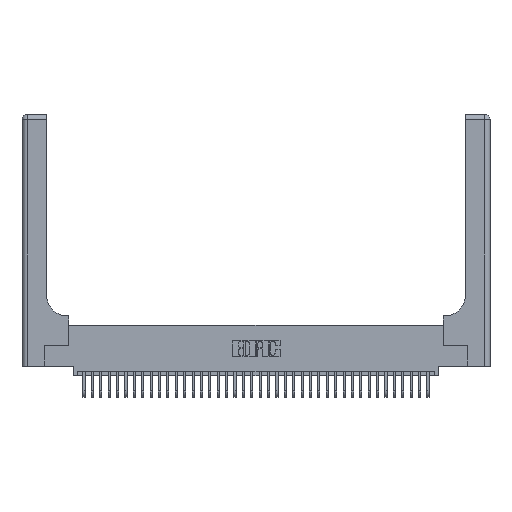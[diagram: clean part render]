
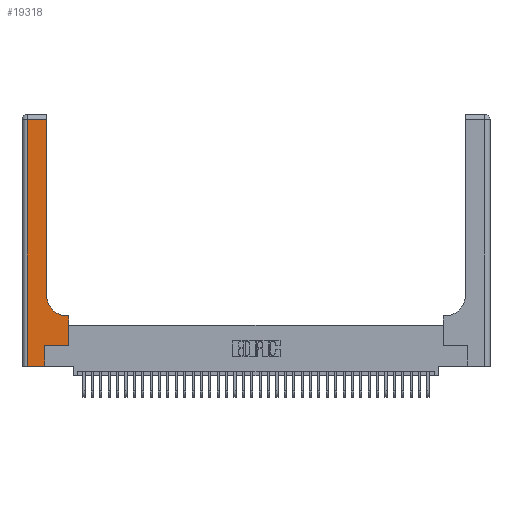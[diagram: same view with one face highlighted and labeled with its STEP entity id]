
A CAD part, top view. The second image highlights one B-rep face of the part: STEP entity #19318.
In plain terms, the highlighted planar face has unit normal (0, 0, 1).
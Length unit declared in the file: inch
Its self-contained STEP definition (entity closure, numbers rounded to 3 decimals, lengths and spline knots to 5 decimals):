
#776 = LINE ( 'NONE', #36630, #22763 ) ;
#889 = VECTOR ( 'NONE', #21785, 39.37008 ) ;
#1633 = VERTEX_POINT ( 'NONE', #10770 ) ;
#1686 = FACE_OUTER_BOUND ( 'NONE', #3178, .T. ) ;
#2050 = ORIENTED_EDGE ( 'NONE', *, *, #23361, .T. ) ;
#2193 = DIRECTION ( 'NONE',  ( -1., 0., 0. ) ) ;
#2312 = DIRECTION ( 'NONE',  ( 0., 0., -1. ) ) ;
#2443 = DIRECTION ( 'NONE',  ( 0., 1., 0. ) ) ;
#2701 = LINE ( 'NONE', #18924, #889 ) ;
#3178 = EDGE_LOOP ( 'NONE', ( #25316, #3786, #7362, #2050, #15601, #27718, #29947, #26872, #20190 ) ) ;
#3778 = VERTEX_POINT ( 'NONE', #33746 ) ;
#3786 = ORIENTED_EDGE ( 'NONE', *, *, #19397, .T. ) ;
#4239 = EDGE_CURVE ( 'NONE', #28799, #34253, #14314, .T. ) ;
#5014 = VERTEX_POINT ( 'NONE', #9779 ) ;
#5049 = CARTESIAN_POINT ( 'NONE',  ( 0.2915, 2.94, 0.37 ) ) ;
#5050 = CARTESIAN_POINT ( 'NONE',  ( 0., 3., 0.37 ) ) ;
#5484 = CARTESIAN_POINT ( 'NONE',  ( 0., 0., 0.37 ) ) ;
#5596 = VERTEX_POINT ( 'NONE', #29403 ) ;
#5608 = VERTEX_POINT ( 'NONE', #12269 ) ;
#7362 = ORIENTED_EDGE ( 'NONE', *, *, #17965, .T. ) ;
#7402 = EDGE_CURVE ( 'NONE', #5014, #5608, #26647, .T. ) ;
#8369 = DIRECTION ( 'NONE',  ( 1., 0., 0. ) ) ;
#8679 = DIRECTION ( 'NONE',  ( 1., 0., 0. ) ) ;
#9344 = DIRECTION ( 'NONE',  ( 0., 1., 0. ) ) ;
#9470 = LINE ( 'NONE', #25890, #30508 ) ;
#9779 = CARTESIAN_POINT ( 'NONE',  ( 0.5585, 0.25, 0.37 ) ) ;
#10365 = DIRECTION ( 'NONE',  ( 0., 1., 0. ) ) ;
#10770 = CARTESIAN_POINT ( 'NONE',  ( 0.5415, 0.6, 0.37 ) ) ;
#11122 = VERTEX_POINT ( 'NONE', #36962 ) ;
#12269 = CARTESIAN_POINT ( 'NONE',  ( 0.5585, 0.6, 0.37 ) ) ;
#13346 = LINE ( 'NONE', #28493, #35201 ) ;
#14314 = LINE ( 'NONE', #21766, #36116 ) ;
#15325 = CARTESIAN_POINT ( 'NONE',  ( 0.5415, 0.85, 0.37 ) ) ;
#15601 = ORIENTED_EDGE ( 'NONE', *, *, #19333, .T. ) ;
#17061 = EDGE_CURVE ( 'NONE', #23232, #5014, #9470, .T. ) ;
#17965 = EDGE_CURVE ( 'NONE', #5596, #11122, #2701, .T. ) ;
#18219 = DIRECTION ( 'NONE',  ( 1., 0., 0. ) ) ;
#18924 = CARTESIAN_POINT ( 'NONE',  ( 0.06, 3., 0.37 ) ) ;
#19011 = VECTOR ( 'NONE', #9344, 39.37008 ) ;
#19014 = LINE ( 'NONE', #30839, #33268 ) ;
#19318 = ADVANCED_FACE ( 'NONE', ( #1686 ), #19497, .F. ) ;
#19333 = EDGE_CURVE ( 'NONE', #3778, #23232, #776, .T. ) ;
#19397 = EDGE_CURVE ( 'NONE', #34253, #5596, #13346, .T. ) ;
#19497 = PLANE ( 'NONE',  #31866 ) ;
#19619 = CARTESIAN_POINT ( 'NONE',  ( 0.2915, 0.85, 0.37 ) ) ;
#20190 = ORIENTED_EDGE ( 'NONE', *, *, #34643, .T. ) ;
#20896 = CARTESIAN_POINT ( 'NONE',  ( 0.5585, 0.25, 0.37 ) ) ;
#21766 = CARTESIAN_POINT ( 'NONE',  ( 0.2915, 3., 0.37 ) ) ;
#21785 = DIRECTION ( 'NONE',  ( 0., -1., 0. ) ) ;
#22364 = DIRECTION ( 'NONE',  ( -1., 0., 0. ) ) ;
#22566 = CIRCLE ( 'NONE', #32774, 0.25 ) ;
#22763 = VECTOR ( 'NONE', #2443, 39.37008 ) ;
#23232 = VERTEX_POINT ( 'NONE', #36202 ) ;
#23361 = EDGE_CURVE ( 'NONE', #11122, #3778, #36904, .T. ) ;
#25316 = ORIENTED_EDGE ( 'NONE', *, *, #4239, .T. ) ;
#25890 = CARTESIAN_POINT ( 'NONE',  ( 0.269, 0.25, 0.37 ) ) ;
#26647 = LINE ( 'NONE', #20896, #19011 ) ;
#26872 = ORIENTED_EDGE ( 'NONE', *, *, #34267, .T. ) ;
#27718 = ORIENTED_EDGE ( 'NONE', *, *, #17061, .T. ) ;
#28493 = CARTESIAN_POINT ( 'NONE',  ( 0., 2.94, 0.37 ) ) ;
#28799 = VERTEX_POINT ( 'NONE', #19619 ) ;
#29403 = CARTESIAN_POINT ( 'NONE',  ( 0.06, 2.94, 0.37 ) ) ;
#29947 = ORIENTED_EDGE ( 'NONE', *, *, #7402, .T. ) ;
#30508 = VECTOR ( 'NONE', #8679, 39.37008 ) ;
#30839 = CARTESIAN_POINT ( 'NONE',  ( 0.2915, 0.6, 0.37 ) ) ;
#31339 = DIRECTION ( 'NONE',  ( -1., 0., 0. ) ) ;
#31866 = AXIS2_PLACEMENT_3D ( 'NONE', #5050, #2312, #22364 ) ;
#32774 = AXIS2_PLACEMENT_3D ( 'NONE', #15325, #35253, #18219 ) ;
#33268 = VECTOR ( 'NONE', #2193, 39.37008 ) ;
#33746 = CARTESIAN_POINT ( 'NONE',  ( 0.269, 0., 0.37 ) ) ;
#34253 = VERTEX_POINT ( 'NONE', #5049 ) ;
#34267 = EDGE_CURVE ( 'NONE', #5608, #1633, #19014, .T. ) ;
#34643 = EDGE_CURVE ( 'NONE', #1633, #28799, #22566, .T. ) ;
#35138 = VECTOR ( 'NONE', #8369, 39.37008 ) ;
#35201 = VECTOR ( 'NONE', #31339, 39.37008 ) ;
#35253 = DIRECTION ( 'NONE',  ( 0., 0., -1. ) ) ;
#36116 = VECTOR ( 'NONE', #10365, 39.37008 ) ;
#36202 = CARTESIAN_POINT ( 'NONE',  ( 0.269, 0.25, 0.37 ) ) ;
#36630 = CARTESIAN_POINT ( 'NONE',  ( 0.269, 0., 0.37 ) ) ;
#36904 = LINE ( 'NONE', #5484, #35138 ) ;
#36962 = CARTESIAN_POINT ( 'NONE',  ( 0.06, 0., 0.37 ) ) ;
